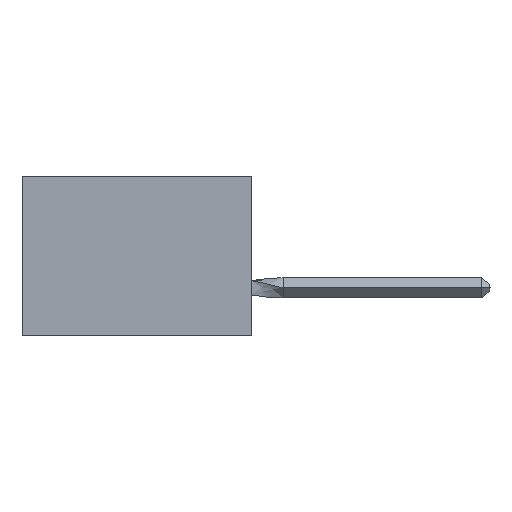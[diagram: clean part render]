
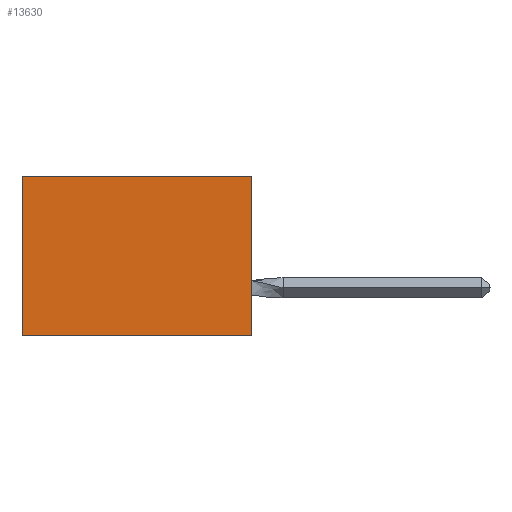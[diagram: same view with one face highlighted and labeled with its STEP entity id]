
A CAD part, left-side view. The second image highlights one B-rep face of the part: STEP entity #13630.
In plain terms, the highlighted planar face has unit normal (-1, 0, 0).
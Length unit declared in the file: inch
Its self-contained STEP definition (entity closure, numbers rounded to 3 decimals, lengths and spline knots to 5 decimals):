
#373 = DIRECTION ( 'NONE',  ( 0., 1., 0. ) ) ;
#1181 = VECTOR ( 'NONE', #8281, 39.37008 ) ;
#2233 = ORIENTED_EDGE ( 'NONE', *, *, #14646, .F. ) ;
#3968 = VECTOR ( 'NONE', #373, 39.37008 ) ;
#5526 = DIRECTION ( 'NONE',  ( 0., 0., -1. ) ) ;
#6499 = EDGE_CURVE ( 'NONE', #8975, #22063, #20634, .T. ) ;
#6870 = FACE_OUTER_BOUND ( 'NONE', #16446, .T. ) ;
#8281 = DIRECTION ( 'NONE',  ( 0., 0., -1. ) ) ;
#8337 = DIRECTION ( 'NONE',  ( 0., 0., -1. ) ) ;
#8975 = VERTEX_POINT ( 'NONE', #11691 ) ;
#9531 = LINE ( 'NONE', #21677, #3968 ) ;
#10168 = EDGE_CURVE ( 'NONE', #23685, #8975, #9531, .T. ) ;
#10928 = EDGE_CURVE ( 'NONE', #26713, #22063, #17498, .T. ) ;
#11298 = AXIS2_PLACEMENT_3D ( 'NONE', #16784, #21223, #8337 ) ;
#11691 = CARTESIAN_POINT ( 'NONE',  ( 0.305, 0.72, 0. ) ) ;
#11962 = CARTESIAN_POINT ( 'NONE',  ( 0.305, 0., -0.5 ) ) ;
#12857 = VECTOR ( 'NONE', #19324, 39.37008 ) ;
#12867 = ORIENTED_EDGE ( 'NONE', *, *, #10928, .F. ) ;
#13104 = LINE ( 'NONE', #13761, #18053 ) ;
#13630 = ADVANCED_FACE ( 'NONE', ( #6870 ), #21124, .F. ) ;
#13761 = CARTESIAN_POINT ( 'NONE',  ( 0.305, 0., -0.5 ) ) ;
#14594 = CARTESIAN_POINT ( 'NONE',  ( 0.305, 0.72, -0.5 ) ) ;
#14646 = EDGE_CURVE ( 'NONE', #23685, #26713, #13104, .T. ) ;
#16039 = ORIENTED_EDGE ( 'NONE', *, *, #10168, .T. ) ;
#16446 = EDGE_LOOP ( 'NONE', ( #23631, #12867, #2233, #16039 ) ) ;
#16784 = CARTESIAN_POINT ( 'NONE',  ( 0.305, 0., -0.5 ) ) ;
#17498 = LINE ( 'NONE', #23720, #12857 ) ;
#18053 = VECTOR ( 'NONE', #5526, 39.37008 ) ;
#19324 = DIRECTION ( 'NONE',  ( 0., 1., 0. ) ) ;
#19731 = CARTESIAN_POINT ( 'NONE',  ( 0.305, 0., 0. ) ) ;
#20634 = LINE ( 'NONE', #14594, #1181 ) ;
#21124 = PLANE ( 'NONE',  #11298 ) ;
#21223 = DIRECTION ( 'NONE',  ( 1., 0., 0. ) ) ;
#21677 = CARTESIAN_POINT ( 'NONE',  ( 0.305, 0., 0. ) ) ;
#22063 = VERTEX_POINT ( 'NONE', #24643 ) ;
#23631 = ORIENTED_EDGE ( 'NONE', *, *, #6499, .T. ) ;
#23685 = VERTEX_POINT ( 'NONE', #19731 ) ;
#23720 = CARTESIAN_POINT ( 'NONE',  ( 0.305, 0., -0.5 ) ) ;
#24643 = CARTESIAN_POINT ( 'NONE',  ( 0.305, 0.72, -0.5 ) ) ;
#26713 = VERTEX_POINT ( 'NONE', #11962 ) ;
